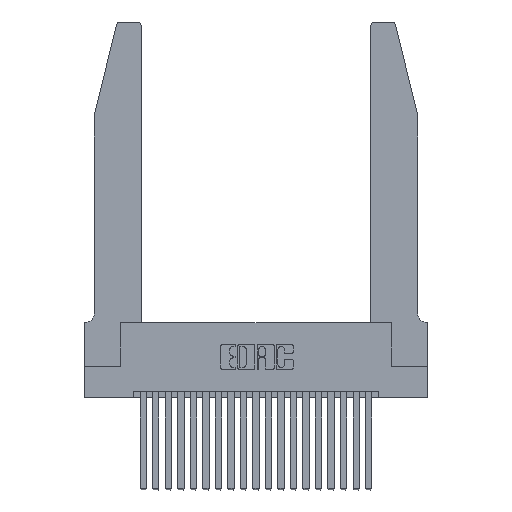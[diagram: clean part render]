
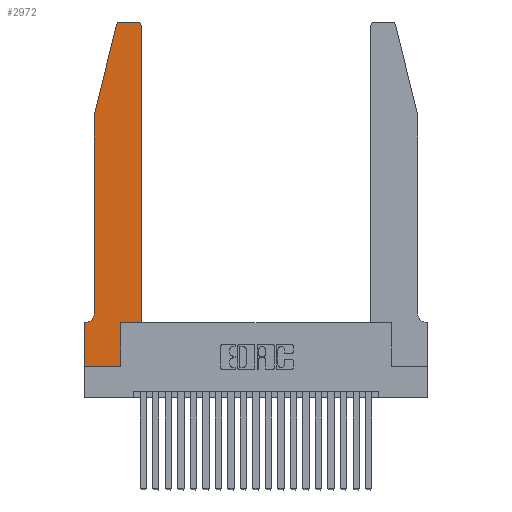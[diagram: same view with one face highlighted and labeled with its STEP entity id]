
A CAD part, top view. The second image highlights one B-rep face of the part: STEP entity #2972.
In plain terms, the highlighted planar face has unit normal (0, 0, 1).
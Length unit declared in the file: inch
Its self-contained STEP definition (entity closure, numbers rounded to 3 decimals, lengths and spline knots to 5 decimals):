
#129 = EDGE_CURVE ( 'NONE', #13087, #4923, #5756, .T. ) ;
#172 = DIRECTION ( 'NONE',  ( 1., 0., 0. ) ) ;
#475 = VERTEX_POINT ( 'NONE', #17408 ) ;
#488 = VECTOR ( 'NONE', #1483, 39.37008 ) ;
#521 = CARTESIAN_POINT ( 'NONE',  ( 0.284, 2.75, 0.37 ) ) ;
#605 = EDGE_CURVE ( 'NONE', #8963, #13277, #1509, .T. ) ;
#1341 = ORIENTED_EDGE ( 'NONE', *, *, #129, .T. ) ;
#1480 = AXIS2_PLACEMENT_3D ( 'NONE', #21096, #10832, #172 ) ;
#1483 = DIRECTION ( 'NONE',  ( 0., 1., 0. ) ) ;
#1509 = LINE ( 'NONE', #1863, #10950 ) ;
#1674 = CARTESIAN_POINT ( 'NONE',  ( 0.0755, 2., 0.37 ) ) ;
#1808 = VERTEX_POINT ( 'NONE', #8070 ) ;
#1863 = CARTESIAN_POINT ( 'NONE',  ( 0., 0., 0.37 ) ) ;
#1950 = DIRECTION ( 'NONE',  ( 0., 0., 1. ) ) ;
#2067 = ORIENTED_EDGE ( 'NONE', *, *, #11787, .T. ) ;
#2213 = DIRECTION ( 'NONE',  ( 1., 0., 0. ) ) ;
#2358 = CARTESIAN_POINT ( 'NONE',  ( 0.25487, 2.72718, 0.37 ) ) ;
#2649 = CARTESIAN_POINT ( 'NONE',  ( 0., 0.35, 0.37 ) ) ;
#2972 = ADVANCED_FACE ( 'NONE', ( #8385 ), #14973, .T. ) ;
#3122 = LINE ( 'NONE', #15970, #12483 ) ;
#3765 = EDGE_CURVE ( 'NONE', #12416, #475, #8623, .T. ) ;
#4295 = ORIENTED_EDGE ( 'NONE', *, *, #18391, .T. ) ;
#4329 = ORIENTED_EDGE ( 'NONE', *, *, #17703, .T. ) ;
#4553 = CARTESIAN_POINT ( 'NONE',  ( 0., 0.35, 0.37 ) ) ;
#4923 = VERTEX_POINT ( 'NONE', #2358 ) ;
#5469 = DIRECTION ( 'NONE',  ( 0., 1., 0. ) ) ;
#5552 = DIRECTION ( 'NONE',  ( -1., 0., 0. ) ) ;
#5581 = VERTEX_POINT ( 'NONE', #9747 ) ;
#5583 = EDGE_CURVE ( 'NONE', #1808, #13087, #15061, .T. ) ;
#5679 = CARTESIAN_POINT ( 'NONE',  ( 0., 0., 0.37 ) ) ;
#5756 = CIRCLE ( 'NONE', #6650, 0.03 ) ;
#6121 = VECTOR ( 'NONE', #5469, 39.37008 ) ;
#6313 = DIRECTION ( 'NONE',  ( 0., 0., 1. ) ) ;
#6650 = AXIS2_PLACEMENT_3D ( 'NONE', #11826, #1950, #2213 ) ;
#6813 = ORIENTED_EDGE ( 'NONE', *, *, #18551, .T. ) ;
#7168 = CARTESIAN_POINT ( 'NONE',  ( 0.2865, 0.35, 0.37 ) ) ;
#7383 = DIRECTION ( 'NONE',  ( 1., 0., 0. ) ) ;
#7470 = CARTESIAN_POINT ( 'NONE',  ( 0.0055, 0.35, 0.37 ) ) ;
#7522 = EDGE_CURVE ( 'NONE', #13277, #15100, #10438, .T. ) ;
#7526 = VECTOR ( 'NONE', #8444, 39.37008 ) ;
#8003 = LINE ( 'NONE', #21343, #21175 ) ;
#8070 = CARTESIAN_POINT ( 'NONE',  ( 0.4205, 2.75, 0.37 ) ) ;
#8385 = FACE_OUTER_BOUND ( 'NONE', #17731, .T. ) ;
#8444 = DIRECTION ( 'NONE',  ( 1., 0., 0. ) ) ;
#8623 = LINE ( 'NONE', #17048, #7526 ) ;
#8669 = ORIENTED_EDGE ( 'NONE', *, *, #605, .T. ) ;
#8704 = DIRECTION ( 'NONE',  ( 0., 0., -1. ) ) ;
#8963 = VERTEX_POINT ( 'NONE', #2649 ) ;
#9747 = CARTESIAN_POINT ( 'NONE',  ( 0.0755, 2., 0.37 ) ) ;
#9848 = CARTESIAN_POINT ( 'NONE',  ( 0., 0., 0.37 ) ) ;
#10438 = LINE ( 'NONE', #5679, #15030 ) ;
#10778 = LINE ( 'NONE', #7168, #6121 ) ;
#10832 = DIRECTION ( 'NONE',  ( 0., 0., 1. ) ) ;
#10950 = VECTOR ( 'NONE', #12679, 39.37008 ) ;
#11086 = ORIENTED_EDGE ( 'NONE', *, *, #18524, .T. ) ;
#11507 = DIRECTION ( 'NONE',  ( -1., 0., 0. ) ) ;
#11787 = EDGE_CURVE ( 'NONE', #18622, #8963, #3122, .T. ) ;
#11826 = CARTESIAN_POINT ( 'NONE',  ( 0.284, 2.72, 0.37 ) ) ;
#12075 = CARTESIAN_POINT ( 'NONE',  ( 0.4505, 0.35, 0.37 ) ) ;
#12370 = EDGE_CURVE ( 'NONE', #5581, #17762, #19421, .T. ) ;
#12416 = VERTEX_POINT ( 'NONE', #14070 ) ;
#12446 = ORIENTED_EDGE ( 'NONE', *, *, #7522, .T. ) ;
#12483 = VECTOR ( 'NONE', #5552, 39.37008 ) ;
#12679 = DIRECTION ( 'NONE',  ( 0., -1., 0. ) ) ;
#13064 = EDGE_CURVE ( 'NONE', #4923, #5581, #8003, .T. ) ;
#13074 = ORIENTED_EDGE ( 'NONE', *, *, #3765, .T. ) ;
#13087 = VERTEX_POINT ( 'NONE', #521 ) ;
#13277 = VERTEX_POINT ( 'NONE', #9848 ) ;
#13739 = AXIS2_PLACEMENT_3D ( 'NONE', #19028, #8704, #20715 ) ;
#14036 = LINE ( 'NONE', #12075, #488 ) ;
#14070 = CARTESIAN_POINT ( 'NONE',  ( 0.2865, 0.35, 0.37 ) ) ;
#14561 = CARTESIAN_POINT ( 'NONE',  ( 0.4505, 2.72, 0.37 ) ) ;
#14880 = VERTEX_POINT ( 'NONE', #14561 ) ;
#14973 = PLANE ( 'NONE',  #20557 ) ;
#15030 = VECTOR ( 'NONE', #7383, 39.37008 ) ;
#15061 = LINE ( 'NONE', #20035, #19091 ) ;
#15100 = VERTEX_POINT ( 'NONE', #21937 ) ;
#15970 = CARTESIAN_POINT ( 'NONE',  ( 0.0755, 0.35, 0.37 ) ) ;
#16685 = ORIENTED_EDGE ( 'NONE', *, *, #12370, .T. ) ;
#17048 = CARTESIAN_POINT ( 'NONE',  ( 0.4505, 0.35, 0.37 ) ) ;
#17408 = CARTESIAN_POINT ( 'NONE',  ( 0.4505, 0.35, 0.37 ) ) ;
#17703 = EDGE_CURVE ( 'NONE', #475, #14880, #14036, .T. ) ;
#17731 = EDGE_LOOP ( 'NONE', ( #20121, #1341, #21798, #16685, #4295, #2067, #8669, #12446, #11086, #13074, #4329, #6813 ) ) ;
#17759 = CIRCLE ( 'NONE', #13739, 0.07 ) ;
#17762 = VERTEX_POINT ( 'NONE', #19054 ) ;
#17939 = DIRECTION ( 'NONE',  ( -0.239, -0.971, 0. ) ) ;
#18391 = EDGE_CURVE ( 'NONE', #17762, #18622, #17759, .T. ) ;
#18447 = DIRECTION ( 'NONE',  ( 1., 0., 0. ) ) ;
#18524 = EDGE_CURVE ( 'NONE', #15100, #12416, #10778, .T. ) ;
#18551 = EDGE_CURVE ( 'NONE', #14880, #1808, #19381, .T. ) ;
#18622 = VERTEX_POINT ( 'NONE', #7470 ) ;
#18884 = VECTOR ( 'NONE', #20771, 39.37008 ) ;
#19028 = CARTESIAN_POINT ( 'NONE',  ( 0.0055, 0.42, 0.37 ) ) ;
#19054 = CARTESIAN_POINT ( 'NONE',  ( 0.0755, 0.42, 0.37 ) ) ;
#19091 = VECTOR ( 'NONE', #11507, 39.37008 ) ;
#19381 = CIRCLE ( 'NONE', #1480, 0.03 ) ;
#19421 = LINE ( 'NONE', #1674, #18884 ) ;
#20035 = CARTESIAN_POINT ( 'NONE',  ( 0.2605, 2.75, 0.37 ) ) ;
#20121 = ORIENTED_EDGE ( 'NONE', *, *, #5583, .T. ) ;
#20557 = AXIS2_PLACEMENT_3D ( 'NONE', #4553, #6313, #18447 ) ;
#20715 = DIRECTION ( 'NONE',  ( -1., 0., 0. ) ) ;
#20771 = DIRECTION ( 'NONE',  ( 0., -1., 0. ) ) ;
#21096 = CARTESIAN_POINT ( 'NONE',  ( 0.4205, 2.72, 0.37 ) ) ;
#21175 = VECTOR ( 'NONE', #17939, 39.37008 ) ;
#21343 = CARTESIAN_POINT ( 'NONE',  ( 0.0755, 2., 0.37 ) ) ;
#21798 = ORIENTED_EDGE ( 'NONE', *, *, #13064, .T. ) ;
#21937 = CARTESIAN_POINT ( 'NONE',  ( 0.2865, 0., 0.37 ) ) ;
